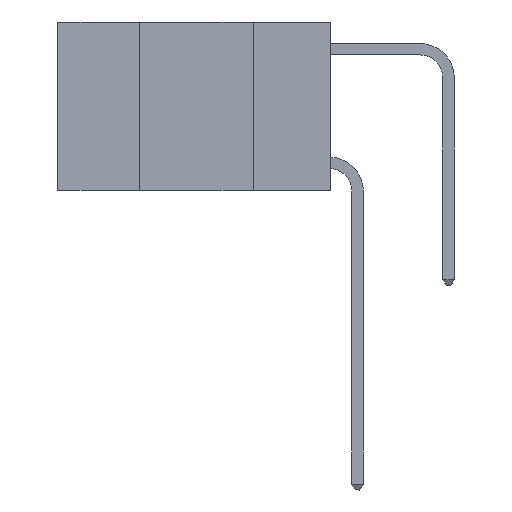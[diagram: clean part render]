
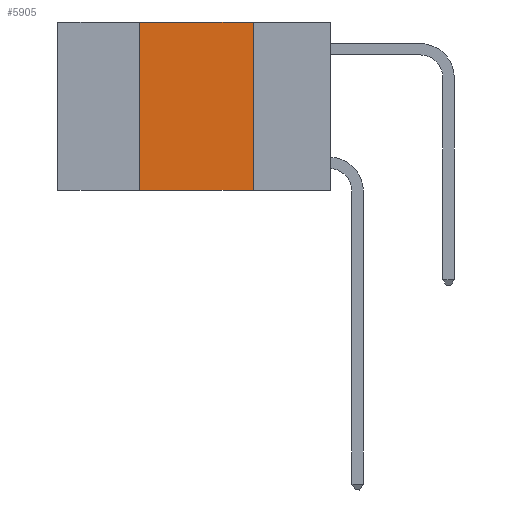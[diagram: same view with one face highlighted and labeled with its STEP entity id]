
A CAD part, left-side view. The second image highlights one B-rep face of the part: STEP entity #5905.
In plain terms, the highlighted planar face has unit normal (-1, 0, 0).
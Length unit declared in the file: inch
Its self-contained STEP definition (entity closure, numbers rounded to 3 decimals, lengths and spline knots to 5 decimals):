
#340 = PLANE ( 'NONE',  #13542 ) ;
#352 = ORIENTED_EDGE ( 'NONE', *, *, #19233, .F. ) ;
#650 = DIRECTION ( 'NONE',  ( 0., 0., -1. ) ) ;
#1381 = EDGE_CURVE ( 'NONE', #20476, #2619, #20725, .T. ) ;
#1919 = LINE ( 'NONE', #7396, #19669 ) ;
#2619 = VERTEX_POINT ( 'NONE', #11479 ) ;
#3031 = DIRECTION ( 'NONE',  ( 0., -1., 0. ) ) ;
#3496 = CARTESIAN_POINT ( 'NONE',  ( 0., 0.42, -0.37 ) ) ;
#3700 = EDGE_CURVE ( 'NONE', #6985, #2619, #14484, .T. ) ;
#3836 = DIRECTION ( 'NONE',  ( 0., 0., -1. ) ) ;
#5905 = ADVANCED_FACE ( 'NONE', ( #14402 ), #340, .F. ) ;
#6432 = EDGE_LOOP ( 'NONE', ( #22198, #352, #18243, #18866 ) ) ;
#6985 = VERTEX_POINT ( 'NONE', #3496 ) ;
#7229 = DIRECTION ( 'NONE',  ( 0., -1., 0. ) ) ;
#7396 = CARTESIAN_POINT ( 'NONE',  ( 0., 0.42, 0. ) ) ;
#8389 = VECTOR ( 'NONE', #7229, 39.37008 ) ;
#10900 = DIRECTION ( 'NONE',  ( 0., 0., 1. ) ) ;
#10978 = CARTESIAN_POINT ( 'NONE',  ( 0., 0.17, 0. ) ) ;
#11479 = CARTESIAN_POINT ( 'NONE',  ( 0., 0.17, -0.37 ) ) ;
#12340 = CARTESIAN_POINT ( 'NONE',  ( 0., 0.6, 0. ) ) ;
#12366 = CARTESIAN_POINT ( 'NONE',  ( 0., 0.17, 0. ) ) ;
#12426 = CARTESIAN_POINT ( 'NONE',  ( 0., 0.6, 0. ) ) ;
#13352 = CARTESIAN_POINT ( 'NONE',  ( 0., 0.6, -0.37 ) ) ;
#13542 = AXIS2_PLACEMENT_3D ( 'NONE', #12426, #14175, #3836 ) ;
#13962 = VECTOR ( 'NONE', #3031, 39.37008 ) ;
#14175 = DIRECTION ( 'NONE',  ( 1., 0., 0. ) ) ;
#14402 = FACE_OUTER_BOUND ( 'NONE', #6432, .T. ) ;
#14484 = LINE ( 'NONE', #13352, #13962 ) ;
#15412 = VERTEX_POINT ( 'NONE', #15796 ) ;
#15796 = CARTESIAN_POINT ( 'NONE',  ( 0., 0.42, 0. ) ) ;
#16758 = VECTOR ( 'NONE', #650, 39.37008 ) ;
#17528 = LINE ( 'NONE', #12340, #8389 ) ;
#18243 = ORIENTED_EDGE ( 'NONE', *, *, #18684, .F. ) ;
#18684 = EDGE_CURVE ( 'NONE', #6985, #15412, #1919, .T. ) ;
#18866 = ORIENTED_EDGE ( 'NONE', *, *, #3700, .T. ) ;
#19233 = EDGE_CURVE ( 'NONE', #15412, #20476, #17528, .T. ) ;
#19669 = VECTOR ( 'NONE', #10900, 39.37008 ) ;
#20476 = VERTEX_POINT ( 'NONE', #12366 ) ;
#20725 = LINE ( 'NONE', #10978, #16758 ) ;
#22198 = ORIENTED_EDGE ( 'NONE', *, *, #1381, .F. ) ;
